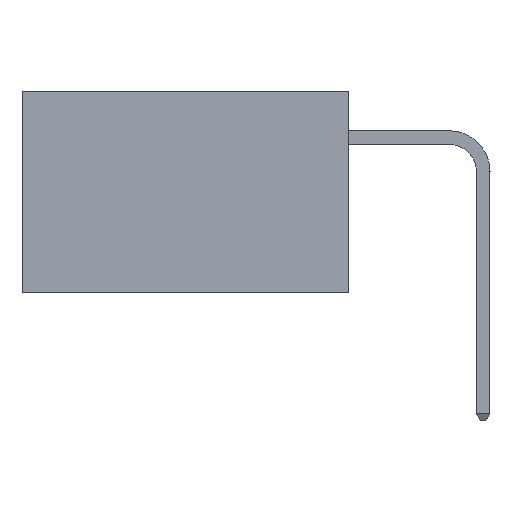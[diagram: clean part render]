
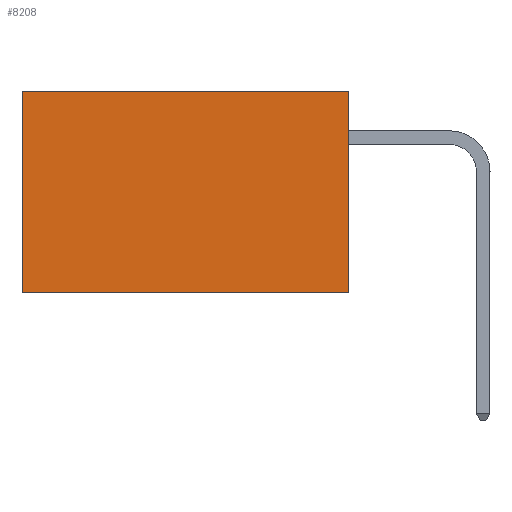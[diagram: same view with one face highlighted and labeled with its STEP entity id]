
A CAD part, left-side view. The second image highlights one B-rep face of the part: STEP entity #8208.
In plain terms, the highlighted planar face has unit normal (-1, 0, 0).
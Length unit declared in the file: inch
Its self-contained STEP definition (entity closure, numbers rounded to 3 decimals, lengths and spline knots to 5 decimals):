
#286 = EDGE_LOOP ( 'NONE', ( #13720, #12897, #22818, #15711 ) ) ;
#1723 = VECTOR ( 'NONE', #4872, 39.37008 ) ;
#3478 = LINE ( 'NONE', #4362, #22130 ) ;
#3714 = LINE ( 'NONE', #13880, #12973 ) ;
#4337 = LINE ( 'NONE', #23203, #17697 ) ;
#4362 = CARTESIAN_POINT ( 'NONE',  ( 0.2875, 0.6, 0. ) ) ;
#4872 = DIRECTION ( 'NONE',  ( 0., 0., -1. ) ) ;
#5654 = VERTEX_POINT ( 'NONE', #14087 ) ;
#6025 = EDGE_CURVE ( 'NONE', #5654, #7995, #3478, .T. ) ;
#7995 = VERTEX_POINT ( 'NONE', #16954 ) ;
#8208 = ADVANCED_FACE ( 'NONE', ( #19323 ), #10232, .F. ) ;
#8446 = DIRECTION ( 'NONE',  ( 0., 0., -1. ) ) ;
#9023 = VERTEX_POINT ( 'NONE', #19556 ) ;
#10232 = PLANE ( 'NONE',  #12703 ) ;
#10940 = DIRECTION ( 'NONE',  ( 0., 1., 0. ) ) ;
#11346 = VERTEX_POINT ( 'NONE', #20204 ) ;
#12703 = AXIS2_PLACEMENT_3D ( 'NONE', #15630, #19144, #8446 ) ;
#12897 = ORIENTED_EDGE ( 'NONE', *, *, #21817, .F. ) ;
#12973 = VECTOR ( 'NONE', #15693, 39.37008 ) ;
#13720 = ORIENTED_EDGE ( 'NONE', *, *, #6025, .T. ) ;
#13880 = CARTESIAN_POINT ( 'NONE',  ( 0.2875, 0., -0.37 ) ) ;
#14020 = CARTESIAN_POINT ( 'NONE',  ( 0.2875, 0., 0. ) ) ;
#14087 = CARTESIAN_POINT ( 'NONE',  ( 0.2875, 0.6, 0. ) ) ;
#15630 = CARTESIAN_POINT ( 'NONE',  ( 0.2875, 0., 0. ) ) ;
#15682 = EDGE_CURVE ( 'NONE', #11346, #9023, #16364, .T. ) ;
#15693 = DIRECTION ( 'NONE',  ( 0., 1., 0. ) ) ;
#15711 = ORIENTED_EDGE ( 'NONE', *, *, #21379, .T. ) ;
#16364 = LINE ( 'NONE', #14020, #1723 ) ;
#16954 = CARTESIAN_POINT ( 'NONE',  ( 0.2875, 0.6, -0.37 ) ) ;
#17697 = VECTOR ( 'NONE', #10940, 39.37008 ) ;
#19144 = DIRECTION ( 'NONE',  ( 1., 0., 0. ) ) ;
#19323 = FACE_OUTER_BOUND ( 'NONE', #286, .T. ) ;
#19556 = CARTESIAN_POINT ( 'NONE',  ( 0.2875, 0., -0.37 ) ) ;
#20204 = CARTESIAN_POINT ( 'NONE',  ( 0.2875, 0., 0. ) ) ;
#21379 = EDGE_CURVE ( 'NONE', #11346, #5654, #4337, .T. ) ;
#21817 = EDGE_CURVE ( 'NONE', #9023, #7995, #3714, .T. ) ;
#22130 = VECTOR ( 'NONE', #22400, 39.37008 ) ;
#22400 = DIRECTION ( 'NONE',  ( 0., 0., -1. ) ) ;
#22818 = ORIENTED_EDGE ( 'NONE', *, *, #15682, .F. ) ;
#23203 = CARTESIAN_POINT ( 'NONE',  ( 0.2875, 0., 0. ) ) ;
